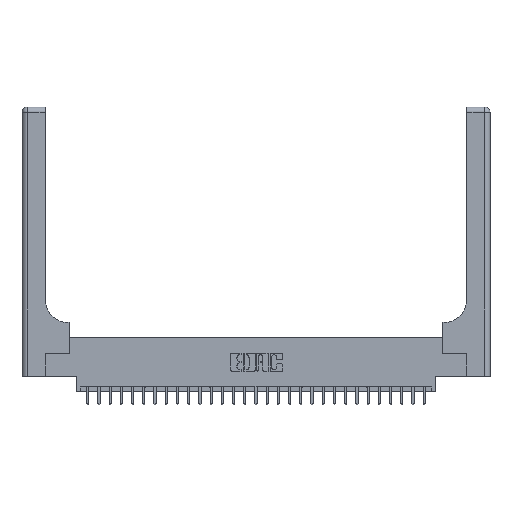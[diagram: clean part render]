
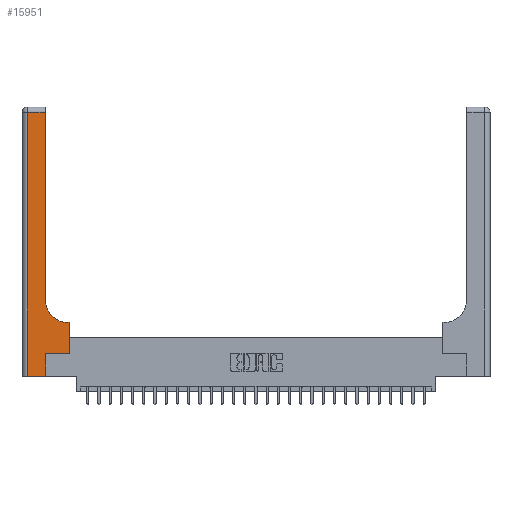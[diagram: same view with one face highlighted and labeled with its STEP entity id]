
A CAD part, top view. The second image highlights one B-rep face of the part: STEP entity #15951.
In plain terms, the highlighted planar face has unit normal (0, 0, 1).
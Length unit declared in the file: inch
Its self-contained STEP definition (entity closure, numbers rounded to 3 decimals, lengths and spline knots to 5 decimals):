
#682 = VERTEX_POINT ( 'NONE', #4425 ) ;
#898 = DIRECTION ( 'NONE',  ( 0., 1., 0. ) ) ;
#1261 = FACE_OUTER_BOUND ( 'NONE', #15531, .T. ) ;
#1458 = LINE ( 'NONE', #7138, #11042 ) ;
#1508 = VECTOR ( 'NONE', #22374, 39.37008 ) ;
#1644 = LINE ( 'NONE', #25022, #1508 ) ;
#1814 = CARTESIAN_POINT ( 'NONE',  ( 0.528, 0.25, 0.37 ) ) ;
#2720 = VECTOR ( 'NONE', #8649, 39.37008 ) ;
#3080 = CARTESIAN_POINT ( 'NONE',  ( 0.26, 0.6, 0.37 ) ) ;
#3312 = VECTOR ( 'NONE', #12274, 39.37008 ) ;
#3903 = ORIENTED_EDGE ( 'NONE', *, *, #21212, .T. ) ;
#4425 = CARTESIAN_POINT ( 'NONE',  ( 0.06, 2.94, 0.37 ) ) ;
#5310 = ORIENTED_EDGE ( 'NONE', *, *, #15681, .T. ) ;
#5949 = LINE ( 'NONE', #8186, #9413 ) ;
#6272 = LINE ( 'NONE', #16851, #25374 ) ;
#6306 = EDGE_CURVE ( 'NONE', #17487, #682, #1644, .T. ) ;
#6620 = VECTOR ( 'NONE', #16878, 39.37008 ) ;
#6925 = CARTESIAN_POINT ( 'NONE',  ( 0.26, 2.94, 0.37 ) ) ;
#7138 = CARTESIAN_POINT ( 'NONE',  ( 0.528, 0.25, 0.37 ) ) ;
#7209 = CARTESIAN_POINT ( 'NONE',  ( 0.51, 0.6, 0.37 ) ) ;
#8186 = CARTESIAN_POINT ( 'NONE',  ( 0.265, 0., 0.37 ) ) ;
#8328 = VERTEX_POINT ( 'NONE', #10410 ) ;
#8649 = DIRECTION ( 'NONE',  ( 1., 0., 0. ) ) ;
#8801 = VECTOR ( 'NONE', #20458, 39.37008 ) ;
#9413 = VECTOR ( 'NONE', #16939, 39.37008 ) ;
#10410 = CARTESIAN_POINT ( 'NONE',  ( 0.06, 0., 0.37 ) ) ;
#10633 = CARTESIAN_POINT ( 'NONE',  ( 0.06, 3., 0.37 ) ) ;
#10770 = VERTEX_POINT ( 'NONE', #1814 ) ;
#10852 = EDGE_CURVE ( 'NONE', #12153, #17487, #14201, .T. ) ;
#10879 = DIRECTION ( 'NONE',  ( 1., 0., 0. ) ) ;
#11042 = VECTOR ( 'NONE', #898, 39.37008 ) ;
#12153 = VERTEX_POINT ( 'NONE', #19772 ) ;
#12274 = DIRECTION ( 'NONE',  ( 0., 1., 0. ) ) ;
#12277 = DIRECTION ( 'NONE',  ( 0., 0., -1. ) ) ;
#13115 = LINE ( 'NONE', #19070, #2720 ) ;
#13293 = EDGE_CURVE ( 'NONE', #682, #8328, #25117, .T. ) ;
#13667 = LINE ( 'NONE', #3080, #8801 ) ;
#14070 = DIRECTION ( 'NONE',  ( -1., 0., 0. ) ) ;
#14178 = DIRECTION ( 'NONE',  ( 0., 0., -1. ) ) ;
#14201 = LINE ( 'NONE', #22682, #3312 ) ;
#14477 = CARTESIAN_POINT ( 'NONE',  ( 0., 3., 0.37 ) ) ;
#15531 = EDGE_LOOP ( 'NONE', ( #15790, #16262, #21358, #5310, #26468, #15982, #24772, #3903, #16244 ) ) ;
#15608 = AXIS2_PLACEMENT_3D ( 'NONE', #14477, #12277, #14070 ) ;
#15627 = EDGE_CURVE ( 'NONE', #26748, #10770, #6272, .T. ) ;
#15681 = EDGE_CURVE ( 'NONE', #8328, #22358, #13115, .T. ) ;
#15790 = ORIENTED_EDGE ( 'NONE', *, *, #10852, .T. ) ;
#15951 = ADVANCED_FACE ( 'NONE', ( #1261 ), #20579, .F. ) ;
#15982 = ORIENTED_EDGE ( 'NONE', *, *, #15627, .T. ) ;
#16244 = ORIENTED_EDGE ( 'NONE', *, *, #23789, .T. ) ;
#16262 = ORIENTED_EDGE ( 'NONE', *, *, #6306, .T. ) ;
#16851 = CARTESIAN_POINT ( 'NONE',  ( 0.265, 0.25, 0.37 ) ) ;
#16878 = DIRECTION ( 'NONE',  ( 0., -1., 0. ) ) ;
#16939 = DIRECTION ( 'NONE',  ( 0., 1., 0. ) ) ;
#17487 = VERTEX_POINT ( 'NONE', #6925 ) ;
#18737 = CARTESIAN_POINT ( 'NONE',  ( 0.51, 0.85, 0.37 ) ) ;
#19070 = CARTESIAN_POINT ( 'NONE',  ( 0., 0., 0.37 ) ) ;
#19772 = CARTESIAN_POINT ( 'NONE',  ( 0.26, 0.85, 0.37 ) ) ;
#19970 = AXIS2_PLACEMENT_3D ( 'NONE', #18737, #14178, #20967 ) ;
#20458 = DIRECTION ( 'NONE',  ( -1., 0., 0. ) ) ;
#20461 = CARTESIAN_POINT ( 'NONE',  ( 0.265, 0., 0.37 ) ) ;
#20579 = PLANE ( 'NONE',  #15608 ) ;
#20967 = DIRECTION ( 'NONE',  ( 1., 0., 0. ) ) ;
#21212 = EDGE_CURVE ( 'NONE', #26946, #22819, #13667, .T. ) ;
#21358 = ORIENTED_EDGE ( 'NONE', *, *, #13293, .T. ) ;
#21770 = CIRCLE ( 'NONE', #19970, 0.25 ) ;
#21825 = EDGE_CURVE ( 'NONE', #10770, #26946, #1458, .T. ) ;
#22358 = VERTEX_POINT ( 'NONE', #20461 ) ;
#22374 = DIRECTION ( 'NONE',  ( -1., 0., 0. ) ) ;
#22682 = CARTESIAN_POINT ( 'NONE',  ( 0.26, 3., 0.37 ) ) ;
#22819 = VERTEX_POINT ( 'NONE', #7209 ) ;
#23789 = EDGE_CURVE ( 'NONE', #22819, #12153, #21770, .T. ) ;
#24772 = ORIENTED_EDGE ( 'NONE', *, *, #21825, .T. ) ;
#25022 = CARTESIAN_POINT ( 'NONE',  ( 0., 2.94, 0.37 ) ) ;
#25117 = LINE ( 'NONE', #10633, #6620 ) ;
#25136 = CARTESIAN_POINT ( 'NONE',  ( 0.265, 0.25, 0.37 ) ) ;
#25374 = VECTOR ( 'NONE', #10879, 39.37008 ) ;
#25809 = CARTESIAN_POINT ( 'NONE',  ( 0.528, 0.6, 0.37 ) ) ;
#26346 = EDGE_CURVE ( 'NONE', #22358, #26748, #5949, .T. ) ;
#26468 = ORIENTED_EDGE ( 'NONE', *, *, #26346, .T. ) ;
#26748 = VERTEX_POINT ( 'NONE', #25136 ) ;
#26946 = VERTEX_POINT ( 'NONE', #25809 ) ;
